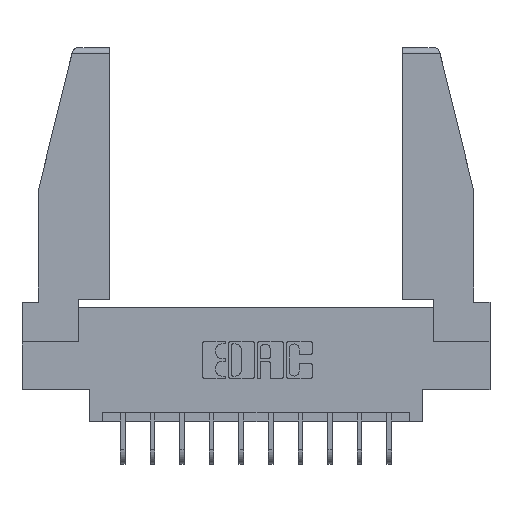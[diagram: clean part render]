
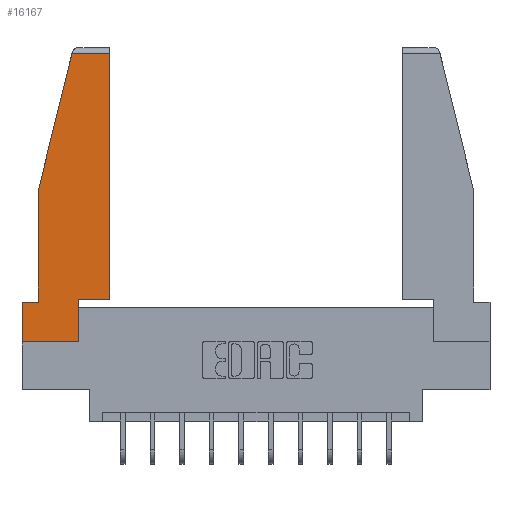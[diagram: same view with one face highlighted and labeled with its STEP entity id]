
A CAD part, top view. The second image highlights one B-rep face of the part: STEP entity #16167.
In plain terms, the highlighted planar face has unit normal (0, 0, 1).
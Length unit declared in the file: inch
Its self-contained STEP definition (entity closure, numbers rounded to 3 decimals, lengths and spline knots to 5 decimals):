
#622 = CARTESIAN_POINT ( 'NONE',  ( 0., 1.52, 0. ) ) ;
#1075 = VECTOR ( 'NONE', #2896, 39.37008 ) ;
#1489 = CARTESIAN_POINT ( 'NONE',  ( 0.297, 0.223, 0. ) ) ;
#1815 = VECTOR ( 'NONE', #14182, 39.37008 ) ;
#2407 = CARTESIAN_POINT ( 'NONE',  ( 0.461, 1.52, 0. ) ) ;
#2483 = EDGE_LOOP ( 'NONE', ( #12214, #4536, #13009, #7864, #5105, #5929, #13119, #14703, #8597 ) ) ;
#2517 = VECTOR ( 'NONE', #15341, 39.37008 ) ;
#2896 = DIRECTION ( 'NONE',  ( 1., 0., 0. ) ) ;
#3043 = VECTOR ( 'NONE', #15573, 39.37008 ) ;
#3469 = EDGE_CURVE ( 'NONE', #15182, #15531, #12468, .T. ) ;
#3775 = VERTEX_POINT ( 'NONE', #2407 ) ;
#3848 = VERTEX_POINT ( 'NONE', #11264 ) ;
#3853 = LINE ( 'NONE', #13188, #3043 ) ;
#3911 = CARTESIAN_POINT ( 'NONE',  ( 0., 0.21, 0. ) ) ;
#4053 = CARTESIAN_POINT ( 'NONE',  ( 0.2636, 1.52, 0. ) ) ;
#4378 = VERTEX_POINT ( 'NONE', #6224 ) ;
#4528 = VERTEX_POINT ( 'NONE', #10829 ) ;
#4530 = DIRECTION ( 'NONE',  ( 0., 1., 0. ) ) ;
#4536 = ORIENTED_EDGE ( 'NONE', *, *, #13752, .T. ) ;
#4772 = VECTOR ( 'NONE', #16219, 39.37008 ) ;
#4913 = VERTEX_POINT ( 'NONE', #3911 ) ;
#5105 = ORIENTED_EDGE ( 'NONE', *, *, #11561, .T. ) ;
#5205 = CARTESIAN_POINT ( 'NONE',  ( 0.271, 1.55, 0. ) ) ;
#5277 = LINE ( 'NONE', #5205, #13556 ) ;
#5403 = LINE ( 'NONE', #622, #10521 ) ;
#5474 = EDGE_CURVE ( 'NONE', #5922, #3848, #5277, .T. ) ;
#5605 = CARTESIAN_POINT ( 'NONE',  ( 0.297, 0., 0. ) ) ;
#5922 = VERTEX_POINT ( 'NONE', #4053 ) ;
#5929 = ORIENTED_EDGE ( 'NONE', *, *, #7693, .T. ) ;
#6023 = VECTOR ( 'NONE', #13581, 39.37008 ) ;
#6036 = CARTESIAN_POINT ( 'NONE',  ( 0., 0., 0. ) ) ;
#6224 = CARTESIAN_POINT ( 'NONE',  ( 0.086, 0.21, 0. ) ) ;
#6400 = CARTESIAN_POINT ( 'NONE',  ( 0.086, 0.8, 0. ) ) ;
#6487 = CARTESIAN_POINT ( 'NONE',  ( 0.461, 0.223, 0. ) ) ;
#6618 = LINE ( 'NONE', #9932, #6023 ) ;
#6755 = EDGE_CURVE ( 'NONE', #4528, #3775, #15529, .T. ) ;
#7124 = CARTESIAN_POINT ( 'NONE',  ( 0.297, 0., 0. ) ) ;
#7549 = LINE ( 'NONE', #6036, #4772 ) ;
#7693 = EDGE_CURVE ( 'NONE', #4913, #15727, #3853, .T. ) ;
#7835 = DIRECTION ( 'NONE',  ( 1., 0., 0. ) ) ;
#7860 = CARTESIAN_POINT ( 'NONE',  ( 0.297, 0.223, 0. ) ) ;
#7864 = ORIENTED_EDGE ( 'NONE', *, *, #16113, .T. ) ;
#8597 = ORIENTED_EDGE ( 'NONE', *, *, #11312, .T. ) ;
#8946 = PLANE ( 'NONE',  #12176 ) ;
#9053 = DIRECTION ( 'NONE',  ( 0., 0., 1. ) ) ;
#9104 = VECTOR ( 'NONE', #4530, 39.37008 ) ;
#9398 = DIRECTION ( 'NONE',  ( -1., 0., 0. ) ) ;
#9932 = CARTESIAN_POINT ( 'NONE',  ( 0., 0.21, 0. ) ) ;
#10200 = CARTESIAN_POINT ( 'NONE',  ( 0., 0., 0. ) ) ;
#10521 = VECTOR ( 'NONE', #9398, 39.37008 ) ;
#10829 = CARTESIAN_POINT ( 'NONE',  ( 0.461, 0.223, 0. ) ) ;
#11057 = FACE_OUTER_BOUND ( 'NONE', #2483, .T. ) ;
#11250 = LINE ( 'NONE', #6400, #1815 ) ;
#11264 = CARTESIAN_POINT ( 'NONE',  ( 0.086, 0.8, 0. ) ) ;
#11312 = EDGE_CURVE ( 'NONE', #15531, #4528, #12522, .T. ) ;
#11561 = EDGE_CURVE ( 'NONE', #4378, #4913, #6618, .T. ) ;
#12176 = AXIS2_PLACEMENT_3D ( 'NONE', #10200, #9053, #7835 ) ;
#12214 = ORIENTED_EDGE ( 'NONE', *, *, #6755, .T. ) ;
#12468 = LINE ( 'NONE', #7124, #9104 ) ;
#12522 = LINE ( 'NONE', #7860, #1075 ) ;
#13009 = ORIENTED_EDGE ( 'NONE', *, *, #5474, .T. ) ;
#13119 = ORIENTED_EDGE ( 'NONE', *, *, #13938, .T. ) ;
#13188 = CARTESIAN_POINT ( 'NONE',  ( 0., 0.21, 0. ) ) ;
#13351 = CARTESIAN_POINT ( 'NONE',  ( 0., 0., 0. ) ) ;
#13556 = VECTOR ( 'NONE', #15308, 39.37008 ) ;
#13581 = DIRECTION ( 'NONE',  ( -1., 0., 0. ) ) ;
#13752 = EDGE_CURVE ( 'NONE', #3775, #5922, #5403, .T. ) ;
#13938 = EDGE_CURVE ( 'NONE', #15727, #15182, #7549, .T. ) ;
#14182 = DIRECTION ( 'NONE',  ( 0., -1., 0. ) ) ;
#14703 = ORIENTED_EDGE ( 'NONE', *, *, #3469, .T. ) ;
#15182 = VERTEX_POINT ( 'NONE', #5605 ) ;
#15308 = DIRECTION ( 'NONE',  ( -0.239, -0.971, 0. ) ) ;
#15341 = DIRECTION ( 'NONE',  ( 0., 1., 0. ) ) ;
#15529 = LINE ( 'NONE', #6487, #2517 ) ;
#15531 = VERTEX_POINT ( 'NONE', #1489 ) ;
#15573 = DIRECTION ( 'NONE',  ( 0., -1., 0. ) ) ;
#15727 = VERTEX_POINT ( 'NONE', #13351 ) ;
#16113 = EDGE_CURVE ( 'NONE', #3848, #4378, #11250, .T. ) ;
#16167 = ADVANCED_FACE ( 'NONE', ( #11057 ), #8946, .T. ) ;
#16219 = DIRECTION ( 'NONE',  ( 1., 0., 0. ) ) ;
